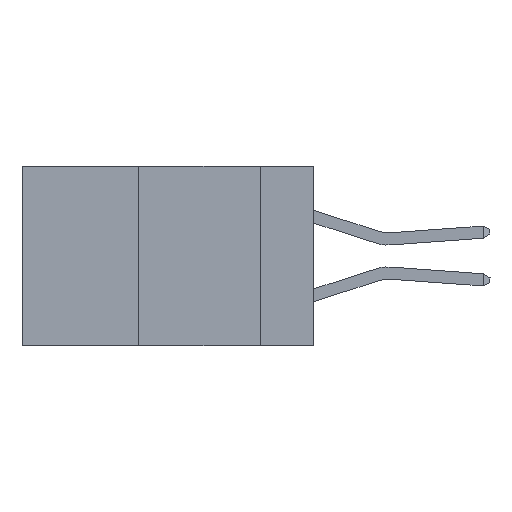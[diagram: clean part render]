
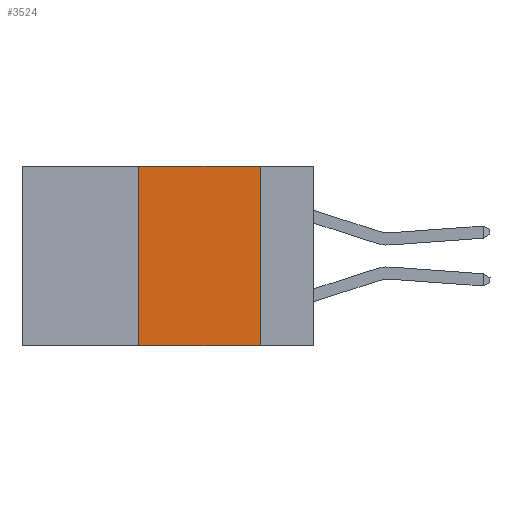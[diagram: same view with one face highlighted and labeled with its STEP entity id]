
A CAD part, left-side view. The second image highlights one B-rep face of the part: STEP entity #3524.
In plain terms, the highlighted planar face has unit normal (-1, 0, 0).
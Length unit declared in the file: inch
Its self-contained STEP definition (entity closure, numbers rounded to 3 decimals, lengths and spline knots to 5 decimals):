
#91 = VERTEX_POINT ( 'NONE', #3594 ) ;
#99 = LINE ( 'NONE', #3434, #5791 ) ;
#155 = CARTESIAN_POINT ( 'NONE',  ( 0., 0.11, 0. ) ) ;
#190 = VERTEX_POINT ( 'NONE', #6717 ) ;
#331 = DIRECTION ( 'NONE',  ( 0., -1., 0. ) ) ;
#1280 = ORIENTED_EDGE ( 'NONE', *, *, #5340, .T. ) ;
#1588 = CARTESIAN_POINT ( 'NONE',  ( 0., 0.11, 0. ) ) ;
#1693 = ORIENTED_EDGE ( 'NONE', *, *, #8701, .F. ) ;
#2022 = LINE ( 'NONE', #155, #9121 ) ;
#2564 = CARTESIAN_POINT ( 'NONE',  ( 0., 0.36, 0. ) ) ;
#2680 = DIRECTION ( 'NONE',  ( 0., 0., -1. ) ) ;
#2993 = DIRECTION ( 'NONE',  ( 1., 0., 0. ) ) ;
#3267 = DIRECTION ( 'NONE',  ( 0., 0., -1. ) ) ;
#3302 = DIRECTION ( 'NONE',  ( 0., -1., 0. ) ) ;
#3434 = CARTESIAN_POINT ( 'NONE',  ( 0., 0.6, -0.37 ) ) ;
#3520 = CARTESIAN_POINT ( 'NONE',  ( 0., 0.36, -0.37 ) ) ;
#3524 = ADVANCED_FACE ( 'NONE', ( #8500 ), #4210, .F. ) ;
#3555 = AXIS2_PLACEMENT_3D ( 'NONE', #4086, #2993, #2680 ) ;
#3594 = CARTESIAN_POINT ( 'NONE',  ( 0., 0.36, 0. ) ) ;
#4086 = CARTESIAN_POINT ( 'NONE',  ( 0., 0.6, 0. ) ) ;
#4210 = PLANE ( 'NONE',  #3555 ) ;
#4215 = DIRECTION ( 'NONE',  ( 0., 0., 1. ) ) ;
#4510 = LINE ( 'NONE', #2564, #7881 ) ;
#4782 = VERTEX_POINT ( 'NONE', #1588 ) ;
#4826 = CARTESIAN_POINT ( 'NONE',  ( 0., 0.6, 0. ) ) ;
#5035 = EDGE_CURVE ( 'NONE', #7324, #91, #4510, .T. ) ;
#5340 = EDGE_CURVE ( 'NONE', #7324, #190, #99, .T. ) ;
#5770 = EDGE_LOOP ( 'NONE', ( #1693, #6663, #7087, #1280 ) ) ;
#5791 = VECTOR ( 'NONE', #3302, 39.37008 ) ;
#6596 = VECTOR ( 'NONE', #331, 39.37008 ) ;
#6663 = ORIENTED_EDGE ( 'NONE', *, *, #8841, .F. ) ;
#6717 = CARTESIAN_POINT ( 'NONE',  ( 0., 0.11, -0.37 ) ) ;
#7087 = ORIENTED_EDGE ( 'NONE', *, *, #5035, .F. ) ;
#7324 = VERTEX_POINT ( 'NONE', #3520 ) ;
#7881 = VECTOR ( 'NONE', #4215, 39.37008 ) ;
#8500 = FACE_OUTER_BOUND ( 'NONE', #5770, .T. ) ;
#8541 = LINE ( 'NONE', #4826, #6596 ) ;
#8701 = EDGE_CURVE ( 'NONE', #4782, #190, #2022, .T. ) ;
#8841 = EDGE_CURVE ( 'NONE', #91, #4782, #8541, .T. ) ;
#9121 = VECTOR ( 'NONE', #3267, 39.37008 ) ;
